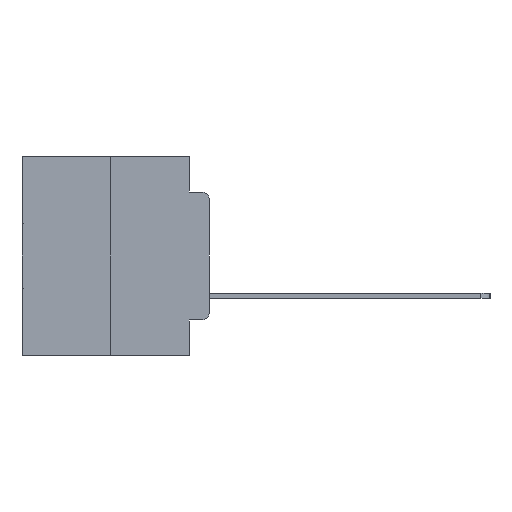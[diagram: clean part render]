
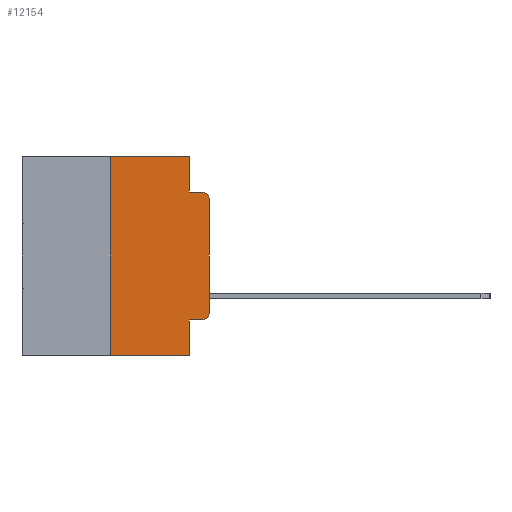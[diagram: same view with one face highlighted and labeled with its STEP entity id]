
A CAD part, left-side view. The second image highlights one B-rep face of the part: STEP entity #12154.
In plain terms, the highlighted planar face has unit normal (-1, 0, 0).
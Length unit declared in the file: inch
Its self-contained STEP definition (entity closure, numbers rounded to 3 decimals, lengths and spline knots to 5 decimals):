
#593 = AXIS2_PLACEMENT_3D ( 'NONE', #19043, #5396, #21271 ) ;
#865 = CARTESIAN_POINT ( 'NONE',  ( 0., 0.25, 0. ) ) ;
#879 = FACE_OUTER_BOUND ( 'NONE', #9095, .T. ) ;
#881 = ORIENTED_EDGE ( 'NONE', *, *, #14201, .F. ) ;
#1090 = EDGE_CURVE ( 'NONE', #17438, #23578, #17081, .T. ) ;
#1486 = VERTEX_POINT ( 'NONE', #17146 ) ;
#1577 = VECTOR ( 'NONE', #13904, 39.37008 ) ;
#2871 = CARTESIAN_POINT ( 'NONE',  ( 0., 0.473, 0. ) ) ;
#3241 = LINE ( 'NONE', #6266, #14705 ) ;
#3374 = VERTEX_POINT ( 'NONE', #23577 ) ;
#3616 = LINE ( 'NONE', #8246, #26964 ) ;
#3722 = DIRECTION ( 'NONE',  ( 0., 0., -1. ) ) ;
#4248 = LINE ( 'NONE', #10751, #21672 ) ;
#5195 = ORIENTED_EDGE ( 'NONE', *, *, #24172, .F. ) ;
#5396 = DIRECTION ( 'NONE',  ( -1., 0., 0. ) ) ;
#6266 = CARTESIAN_POINT ( 'NONE',  ( 0., 0., 0. ) ) ;
#6278 = ORIENTED_EDGE ( 'NONE', *, *, #18636, .T. ) ;
#6281 = LINE ( 'NONE', #865, #28144 ) ;
#7431 = VERTEX_POINT ( 'NONE', #27977 ) ;
#7450 = VERTEX_POINT ( 'NONE', #7762 ) ;
#7480 = DIRECTION ( 'NONE',  ( 0., 0., -1. ) ) ;
#7567 = CARTESIAN_POINT ( 'NONE',  ( 0., 0.02, -0.3915 ) ) ;
#7681 = LINE ( 'NONE', #25069, #1577 ) ;
#7762 = CARTESIAN_POINT ( 'NONE',  ( 0., 0., -0.1085 ) ) ;
#7885 = LINE ( 'NONE', #9434, #13968 ) ;
#8246 = CARTESIAN_POINT ( 'NONE',  ( 0., 0.051, 0. ) ) ;
#8334 = VERTEX_POINT ( 'NONE', #10825 ) ;
#8928 = EDGE_CURVE ( 'NONE', #23578, #7450, #3241, .T. ) ;
#9095 = EDGE_LOOP ( 'NONE', ( #22946, #6278, #18389, #881, #19774, #25692, #21175, #5195, #17361, #18059 ) ) ;
#9434 = CARTESIAN_POINT ( 'NONE',  ( 0., 0.051, -0.4115 ) ) ;
#9565 = CARTESIAN_POINT ( 'NONE',  ( 0., 0.25, 0. ) ) ;
#9572 = EDGE_CURVE ( 'NONE', #12697, #1486, #4248, .T. ) ;
#9692 = PLANE ( 'NONE',  #21330 ) ;
#9782 = CARTESIAN_POINT ( 'NONE',  ( 0., 0.051, -0.0885 ) ) ;
#10243 = VECTOR ( 'NONE', #18885, 39.37008 ) ;
#10751 = CARTESIAN_POINT ( 'NONE',  ( 0., 0.473, 0. ) ) ;
#10825 = CARTESIAN_POINT ( 'NONE',  ( 0., 0.02, -0.0885 ) ) ;
#12154 = ADVANCED_FACE ( 'NONE', ( #879 ), #9692, .F. ) ;
#12535 = CARTESIAN_POINT ( 'NONE',  ( 0., 0.051, -0.4115 ) ) ;
#12697 = VERTEX_POINT ( 'NONE', #9565 ) ;
#12901 = CARTESIAN_POINT ( 'NONE',  ( 0., 0., -0.3915 ) ) ;
#13904 = DIRECTION ( 'NONE',  ( 0., 0., -1. ) ) ;
#13925 = LINE ( 'NONE', #14539, #19211 ) ;
#13968 = VECTOR ( 'NONE', #18545, 39.37008 ) ;
#14201 = EDGE_CURVE ( 'NONE', #1486, #3374, #7681, .T. ) ;
#14539 = CARTESIAN_POINT ( 'NONE',  ( 0., 0.473, -0.5 ) ) ;
#14705 = VECTOR ( 'NONE', #15360, 39.37008 ) ;
#15360 = DIRECTION ( 'NONE',  ( 0., 0., 1. ) ) ;
#16886 = DIRECTION ( 'NONE',  ( 0., 0., 1. ) ) ;
#17081 = CIRCLE ( 'NONE', #28033, 0.02 ) ;
#17146 = CARTESIAN_POINT ( 'NONE',  ( 0., 0.051, 0. ) ) ;
#17361 = ORIENTED_EDGE ( 'NONE', *, *, #26011, .T. ) ;
#17438 = VERTEX_POINT ( 'NONE', #23123 ) ;
#18059 = ORIENTED_EDGE ( 'NONE', *, *, #1090, .T. ) ;
#18389 = ORIENTED_EDGE ( 'NONE', *, *, #22187, .F. ) ;
#18545 = DIRECTION ( 'NONE',  ( 0., -1., 0. ) ) ;
#18588 = DIRECTION ( 'NONE',  ( -1., 0., 0. ) ) ;
#18636 = EDGE_CURVE ( 'NONE', #7450, #8334, #27832, .T. ) ;
#18716 = VERTEX_POINT ( 'NONE', #12535 ) ;
#18885 = DIRECTION ( 'NONE',  ( 0., -1., 0. ) ) ;
#19043 = CARTESIAN_POINT ( 'NONE',  ( 0., 0.02, -0.1085 ) ) ;
#19070 = DIRECTION ( 'NONE',  ( 0., -1., 0. ) ) ;
#19211 = VECTOR ( 'NONE', #19070, 39.37008 ) ;
#19288 = EDGE_CURVE ( 'NONE', #7431, #12697, #6281, .T. ) ;
#19338 = VERTEX_POINT ( 'NONE', #23808 ) ;
#19774 = ORIENTED_EDGE ( 'NONE', *, *, #9572, .F. ) ;
#20375 = EDGE_CURVE ( 'NONE', #7431, #19338, #13925, .T. ) ;
#21039 = DIRECTION ( 'NONE',  ( 1., 0., 0. ) ) ;
#21175 = ORIENTED_EDGE ( 'NONE', *, *, #20375, .T. ) ;
#21271 = DIRECTION ( 'NONE',  ( 0., 0., -1. ) ) ;
#21330 = AXIS2_PLACEMENT_3D ( 'NONE', #2871, #21039, #7480 ) ;
#21672 = VECTOR ( 'NONE', #24321, 39.37008 ) ;
#22187 = EDGE_CURVE ( 'NONE', #3374, #8334, #22960, .T. ) ;
#22946 = ORIENTED_EDGE ( 'NONE', *, *, #8928, .T. ) ;
#22960 = LINE ( 'NONE', #9782, #10243 ) ;
#23123 = CARTESIAN_POINT ( 'NONE',  ( 0., 0.02, -0.4115 ) ) ;
#23577 = CARTESIAN_POINT ( 'NONE',  ( 0., 0.051, -0.0885 ) ) ;
#23578 = VERTEX_POINT ( 'NONE', #12901 ) ;
#23808 = CARTESIAN_POINT ( 'NONE',  ( 0., 0.051, -0.5 ) ) ;
#24172 = EDGE_CURVE ( 'NONE', #18716, #19338, #3616, .T. ) ;
#24321 = DIRECTION ( 'NONE',  ( 0., -1., 0. ) ) ;
#25069 = CARTESIAN_POINT ( 'NONE',  ( 0., 0.051, 0. ) ) ;
#25692 = ORIENTED_EDGE ( 'NONE', *, *, #19288, .F. ) ;
#26011 = EDGE_CURVE ( 'NONE', #18716, #17438, #7885, .T. ) ;
#26092 = DIRECTION ( 'NONE',  ( 0., 0., -1. ) ) ;
#26964 = VECTOR ( 'NONE', #3722, 39.37008 ) ;
#27832 = CIRCLE ( 'NONE', #593, 0.02 ) ;
#27977 = CARTESIAN_POINT ( 'NONE',  ( 0., 0.25, -0.5 ) ) ;
#28033 = AXIS2_PLACEMENT_3D ( 'NONE', #7567, #18588, #26092 ) ;
#28144 = VECTOR ( 'NONE', #16886, 39.37008 ) ;
